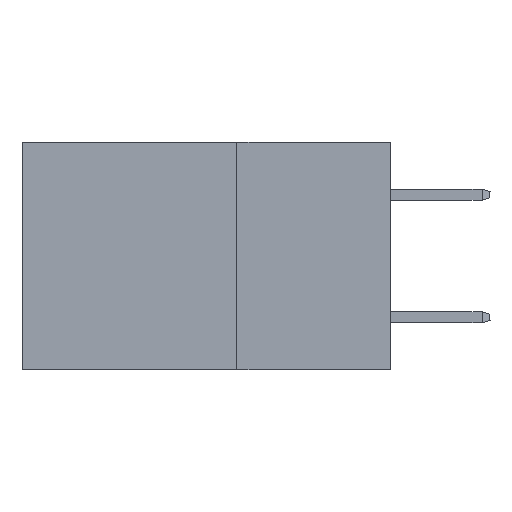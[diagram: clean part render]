
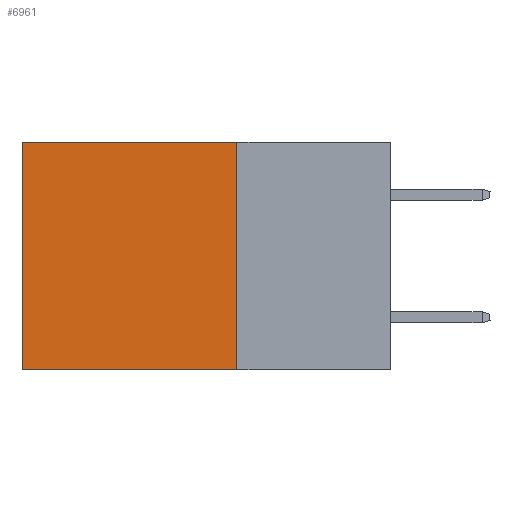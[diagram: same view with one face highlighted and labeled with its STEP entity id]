
A CAD part, left-side view. The second image highlights one B-rep face of the part: STEP entity #6961.
In plain terms, the highlighted planar face has unit normal (-1, 0, 0).
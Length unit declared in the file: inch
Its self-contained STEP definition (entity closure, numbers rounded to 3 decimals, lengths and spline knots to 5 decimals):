
#147 = VERTEX_POINT ( 'NONE', #7213 ) ;
#276 = ORIENTED_EDGE ( 'NONE', *, *, #17201, .F. ) ;
#375 = CARTESIAN_POINT ( 'NONE',  ( 0.2875, 0.6, 0. ) ) ;
#402 = ORIENTED_EDGE ( 'NONE', *, *, #14980, .T. ) ;
#509 = LINE ( 'NONE', #5376, #3699 ) ;
#921 = DIRECTION ( 'NONE',  ( 1., 0., 0. ) ) ;
#2184 = DIRECTION ( 'NONE',  ( 0., 0., -1. ) ) ;
#2422 = VERTEX_POINT ( 'NONE', #8600 ) ;
#3055 = LINE ( 'NONE', #14155, #9411 ) ;
#3699 = VECTOR ( 'NONE', #12829, 39.37008 ) ;
#4424 = EDGE_LOOP ( 'NONE', ( #402, #5320, #276, #14436 ) ) ;
#4486 = FACE_OUTER_BOUND ( 'NONE', #4424, .T. ) ;
#4863 = DIRECTION ( 'NONE',  ( 0., 1., 0. ) ) ;
#5320 = ORIENTED_EDGE ( 'NONE', *, *, #7458, .F. ) ;
#5376 = CARTESIAN_POINT ( 'NONE',  ( 0.2875, 0.25, 0. ) ) ;
#6079 = PLANE ( 'NONE',  #8164 ) ;
#6961 = ADVANCED_FACE ( 'NONE', ( #4486 ), #6079, .F. ) ;
#7213 = CARTESIAN_POINT ( 'NONE',  ( 0.2875, 0.25, 0. ) ) ;
#7398 = LINE ( 'NONE', #375, #12310 ) ;
#7458 = EDGE_CURVE ( 'NONE', #13296, #2422, #8840, .T. ) ;
#8164 = AXIS2_PLACEMENT_3D ( 'NONE', #8372, #921, #10067 ) ;
#8230 = VECTOR ( 'NONE', #4863, 39.37008 ) ;
#8372 = CARTESIAN_POINT ( 'NONE',  ( 0.2875, 0.25, 0. ) ) ;
#8489 = CARTESIAN_POINT ( 'NONE',  ( 0.2875, 0.25, -0.37 ) ) ;
#8600 = CARTESIAN_POINT ( 'NONE',  ( 0.2875, 0.6, -0.37 ) ) ;
#8840 = LINE ( 'NONE', #11996, #8230 ) ;
#9411 = VECTOR ( 'NONE', #16263, 39.37008 ) ;
#10067 = DIRECTION ( 'NONE',  ( 0., 0., -1. ) ) ;
#11996 = CARTESIAN_POINT ( 'NONE',  ( 0.2875, 0.25, -0.37 ) ) ;
#12310 = VECTOR ( 'NONE', #2184, 39.37008 ) ;
#12829 = DIRECTION ( 'NONE',  ( 0., 1., 0. ) ) ;
#13296 = VERTEX_POINT ( 'NONE', #8489 ) ;
#13459 = EDGE_CURVE ( 'NONE', #147, #17809, #509, .T. ) ;
#14155 = CARTESIAN_POINT ( 'NONE',  ( 0.2875, 0.25, 0. ) ) ;
#14259 = CARTESIAN_POINT ( 'NONE',  ( 0.2875, 0.6, 0. ) ) ;
#14436 = ORIENTED_EDGE ( 'NONE', *, *, #13459, .T. ) ;
#14980 = EDGE_CURVE ( 'NONE', #17809, #2422, #7398, .T. ) ;
#16263 = DIRECTION ( 'NONE',  ( 0., 0., -1. ) ) ;
#17201 = EDGE_CURVE ( 'NONE', #147, #13296, #3055, .T. ) ;
#17809 = VERTEX_POINT ( 'NONE', #14259 ) ;
